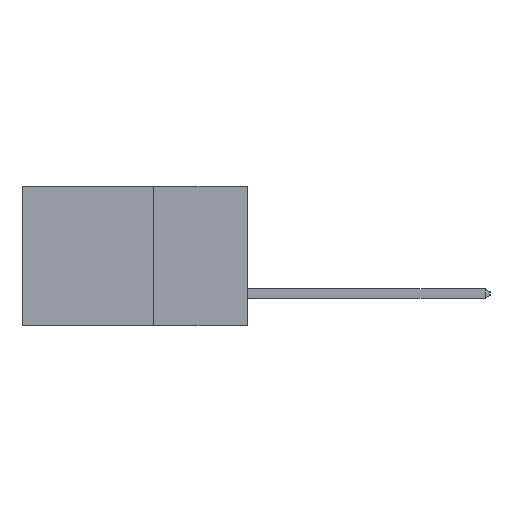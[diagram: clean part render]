
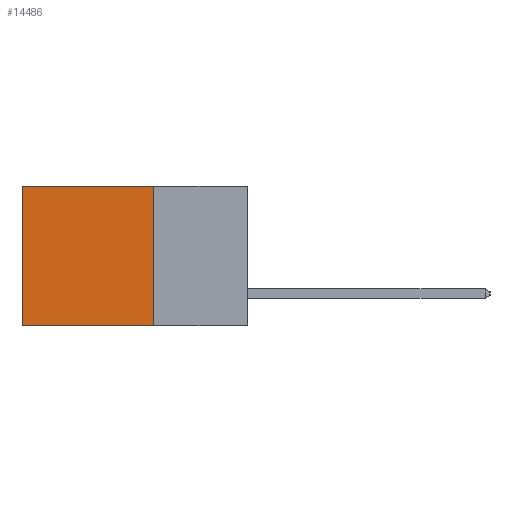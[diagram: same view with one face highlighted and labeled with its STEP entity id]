
A CAD part, left-side view. The second image highlights one B-rep face of the part: STEP entity #14486.
In plain terms, the highlighted planar face has unit normal (-1, 0, 0).
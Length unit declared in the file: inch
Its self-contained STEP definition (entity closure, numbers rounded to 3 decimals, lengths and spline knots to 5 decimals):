
#450 = EDGE_CURVE ( 'NONE', #1392, #17115, #17625, .T. ) ;
#533 = VERTEX_POINT ( 'NONE', #15036 ) ;
#776 = ORIENTED_EDGE ( 'NONE', *, *, #9284, .F. ) ;
#1247 = DIRECTION ( 'NONE',  ( 1., 0., 0. ) ) ;
#1392 = VERTEX_POINT ( 'NONE', #10481 ) ;
#1768 = CARTESIAN_POINT ( 'NONE',  ( 0.298, 0.6, -0.37 ) ) ;
#4002 = CARTESIAN_POINT ( 'NONE',  ( 0.298, 0.6, 0. ) ) ;
#4241 = CARTESIAN_POINT ( 'NONE',  ( 0.298, 0.25, 0. ) ) ;
#5221 = CARTESIAN_POINT ( 'NONE',  ( 0.298, 0.25, 0. ) ) ;
#5466 = ORIENTED_EDGE ( 'NONE', *, *, #450, .F. ) ;
#5704 = PLANE ( 'NONE',  #8673 ) ;
#6241 = VECTOR ( 'NONE', #6946, 39.37008 ) ;
#6613 = EDGE_CURVE ( 'NONE', #18034, #17115, #10536, .T. ) ;
#6946 = DIRECTION ( 'NONE',  ( 0., 0., -1. ) ) ;
#7038 = EDGE_LOOP ( 'NONE', ( #18285, #5466, #776, #14971 ) ) ;
#7090 = DIRECTION ( 'NONE',  ( 0., 0., -1. ) ) ;
#8236 = CARTESIAN_POINT ( 'NONE',  ( 0.298, 0.25, 0. ) ) ;
#8671 = FACE_OUTER_BOUND ( 'NONE', #7038, .T. ) ;
#8673 = AXIS2_PLACEMENT_3D ( 'NONE', #4241, #1247, #7090 ) ;
#9284 = EDGE_CURVE ( 'NONE', #533, #1392, #9577, .T. ) ;
#9577 = LINE ( 'NONE', #5221, #6241 ) ;
#9656 = DIRECTION ( 'NONE',  ( 0., 1., 0. ) ) ;
#10481 = CARTESIAN_POINT ( 'NONE',  ( 0.298, 0.25, -0.37 ) ) ;
#10536 = LINE ( 'NONE', #17230, #17501 ) ;
#11341 = DIRECTION ( 'NONE',  ( 0., 1., 0. ) ) ;
#11464 = CARTESIAN_POINT ( 'NONE',  ( 0.298, 0.25, -0.37 ) ) ;
#13963 = VECTOR ( 'NONE', #11341, 39.37008 ) ;
#14486 = ADVANCED_FACE ( 'NONE', ( #8671 ), #5704, .F. ) ;
#14971 = ORIENTED_EDGE ( 'NONE', *, *, #16794, .T. ) ;
#15036 = CARTESIAN_POINT ( 'NONE',  ( 0.298, 0.25, 0. ) ) ;
#16794 = EDGE_CURVE ( 'NONE', #533, #18034, #17683, .T. ) ;
#17115 = VERTEX_POINT ( 'NONE', #1768 ) ;
#17161 = DIRECTION ( 'NONE',  ( 0., 0., -1. ) ) ;
#17230 = CARTESIAN_POINT ( 'NONE',  ( 0.298, 0.6, 0. ) ) ;
#17257 = VECTOR ( 'NONE', #9656, 39.37008 ) ;
#17501 = VECTOR ( 'NONE', #17161, 39.37008 ) ;
#17625 = LINE ( 'NONE', #11464, #13963 ) ;
#17683 = LINE ( 'NONE', #8236, #17257 ) ;
#18034 = VERTEX_POINT ( 'NONE', #4002 ) ;
#18285 = ORIENTED_EDGE ( 'NONE', *, *, #6613, .T. ) ;
